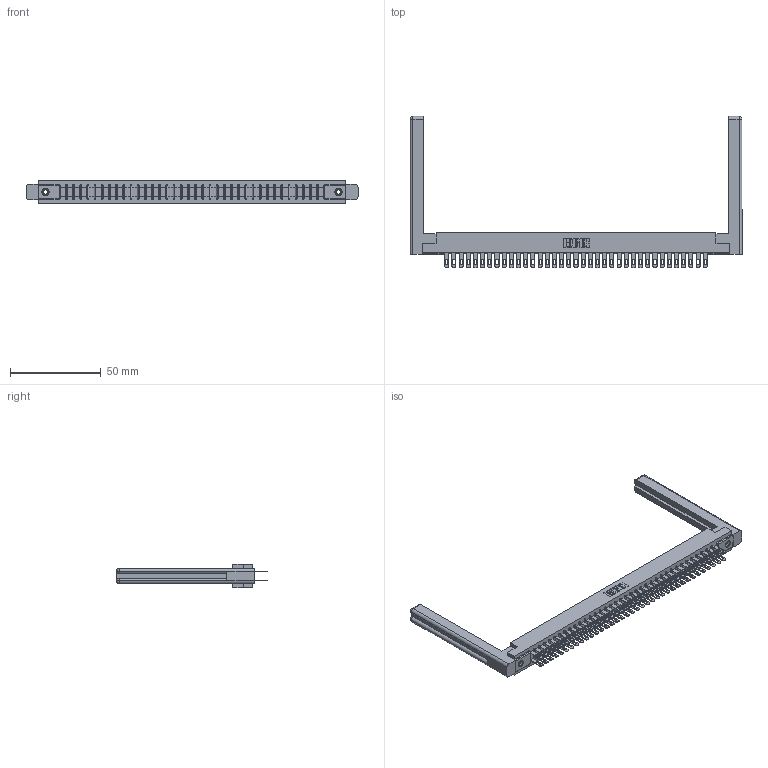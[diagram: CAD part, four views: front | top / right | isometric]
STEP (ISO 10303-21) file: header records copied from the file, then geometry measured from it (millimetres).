
FILE_DESCRIPTION (( 'STEP AP203' ), '1' );
FILE_NAME ('357-074-500-258.STEP', '2019-09-19T12:04:55', ( '' ), ( '' ), 'SwSTEP 2.0', 'SolidWorks 2016', '' );
FILE_SCHEMA (( 'CONFIG_CONTROL_DESIGN' ));
Length unit declared in the file: inch
Products named in the file (5): 357-074-500-258; 345-250-001_345-250-001-102; 307-290-001_500; 307 Part_.156 Dia Mounting Holes; 307-220-058
Assembly tree (79 placements, depth 2):
  357-074-500-258
    307 Part_.156 Dia Mounting Holes
    307-290-001_500  x74
    307-220-058  x2
    345-250-001_345-250-001-102  x2
Bounding box: 183.24 x 83.49 x 12.7 mm (x, y, z)
Volume: 26791 mm3; surface area: 30027.3 mm2
Topology: 79 solids, 79 shells, 3702 faces, 10297 edges, 6650 vertices
Faces by surface type: plane 2374, cylinder 1228, sphere 76, torus 12, cone 12
Entity records: 36127 total; most frequent: CARTESIAN_POINT 5928, ORIENTED_EDGE 5816, DIRECTION 5768, EDGE_CURVE 2908, LINE 2224, VECTOR 2224, VERTEX_POINT 1878, AXIS2_PLACEMENT_3D 1772
